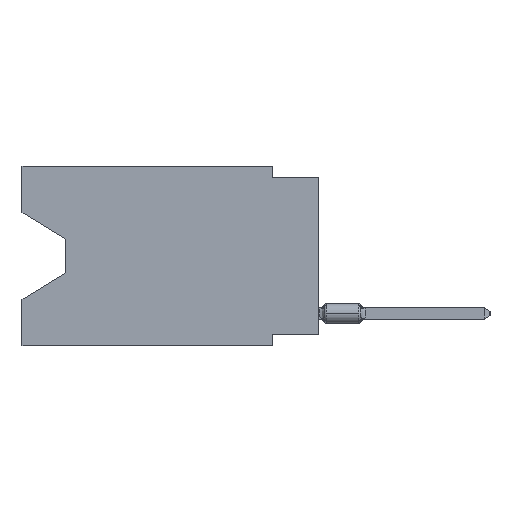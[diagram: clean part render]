
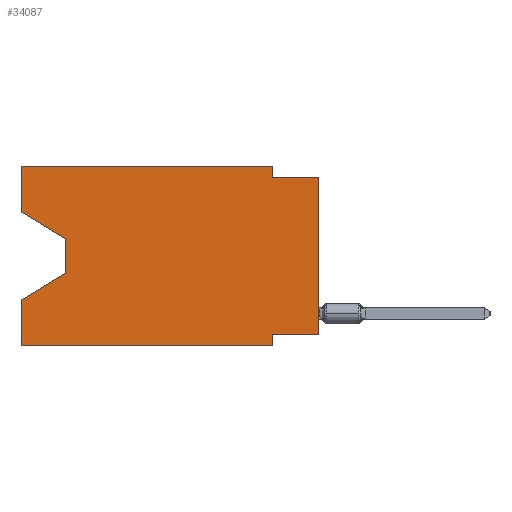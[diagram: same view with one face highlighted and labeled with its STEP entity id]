
A CAD part, left-side view. The second image highlights one B-rep face of the part: STEP entity #34087.
In plain terms, the highlighted planar face has unit normal (-1, 0, 0).
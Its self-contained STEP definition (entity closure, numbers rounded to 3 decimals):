
#524 = VERTEX_POINT ( 'NONE', #874 ) ;
#874 = CARTESIAN_POINT ( 'NONE',  ( 0., 2.54, -9.271 ) ) ;
#1854 = LINE ( 'NONE', #14686, #39917 ) ;
#3191 = FACE_OUTER_BOUND ( 'NONE', #37028, .T. ) ;
#3282 = VERTEX_POINT ( 'NONE', #44641 ) ;
#3413 = CARTESIAN_POINT ( 'NONE',  ( 0., 0., -9.271 ) ) ;
#3425 = VERTEX_POINT ( 'NONE', #6383 ) ;
#3441 = ORIENTED_EDGE ( 'NONE', *, *, #35888, .F. ) ;
#3469 = CARTESIAN_POINT ( 'NONE',  ( 0., 16.383, 0. ) ) ;
#4179 = VECTOR ( 'NONE', #18188, 1000. ) ;
#4365 = ORIENTED_EDGE ( 'NONE', *, *, #12885, .F. ) ;
#5211 = DIRECTION ( 'NONE',  ( 0., 0., 1. ) ) ;
#5479 = CARTESIAN_POINT ( 'NONE',  ( 0., 0., 0. ) ) ;
#5643 = LINE ( 'NONE', #26942, #4179 ) ;
#5719 = ORIENTED_EDGE ( 'NONE', *, *, #15789, .T. ) ;
#6383 = CARTESIAN_POINT ( 'NONE',  ( 0., 16.383, -2.546 ) ) ;
#6594 = ORIENTED_EDGE ( 'NONE', *, *, #8241, .F. ) ;
#6657 = DIRECTION ( 'NONE',  ( 0., 0., -1. ) ) ;
#7640 = CARTESIAN_POINT ( 'NONE',  ( 0., 13.97, -5.893 ) ) ;
#7889 = VECTOR ( 'NONE', #5211, 1000. ) ;
#8241 = EDGE_CURVE ( 'NONE', #13669, #27437, #14014, .T. ) ;
#9284 = VECTOR ( 'NONE', #46920, 1000. ) ;
#10106 = LINE ( 'NONE', #5479, #9284 ) ;
#10117 = LINE ( 'NONE', #22416, #7889 ) ;
#10159 = LINE ( 'NONE', #26845, #22671 ) ;
#10287 = VERTEX_POINT ( 'NONE', #7640 ) ;
#10940 = VECTOR ( 'NONE', #15010, 1000. ) ;
#11008 = ORIENTED_EDGE ( 'NONE', *, *, #31252, .F. ) ;
#11372 = EDGE_CURVE ( 'NONE', #49184, #30886, #10117, .T. ) ;
#11558 = CARTESIAN_POINT ( 'NONE',  ( 0., 2.54, 0. ) ) ;
#11641 = CARTESIAN_POINT ( 'NONE',  ( 0., 2.54, -0.635 ) ) ;
#12885 = EDGE_CURVE ( 'NONE', #27437, #40068, #23904, .T. ) ;
#13579 = CARTESIAN_POINT ( 'NONE',  ( 0., 13.97, -4.013 ) ) ;
#13669 = VERTEX_POINT ( 'NONE', #53870 ) ;
#14014 = LINE ( 'NONE', #11558, #39491 ) ;
#14410 = DIRECTION ( 'NONE',  ( 0., 0.855, -0.519 ) ) ;
#14686 = CARTESIAN_POINT ( 'NONE',  ( 0., 13.97, -5.893 ) ) ;
#15010 = DIRECTION ( 'NONE',  ( 0., -1., 0. ) ) ;
#15322 = EDGE_CURVE ( 'NONE', #33031, #40068, #10106, .T. ) ;
#15789 = EDGE_CURVE ( 'NONE', #10287, #30886, #1854, .T. ) ;
#17598 = ORIENTED_EDGE ( 'NONE', *, *, #26671, .F. ) ;
#17876 = CARTESIAN_POINT ( 'NONE',  ( 0., 0., -9.271 ) ) ;
#18188 = DIRECTION ( 'NONE',  ( 0., 0., 1. ) ) ;
#19279 = DIRECTION ( 'NONE',  ( 0., 1., 0. ) ) ;
#21974 = VECTOR ( 'NONE', #50192, 1000. ) ;
#22416 = CARTESIAN_POINT ( 'NONE',  ( 0., 16.383, 0. ) ) ;
#22671 = VECTOR ( 'NONE', #36095, 1000. ) ;
#22912 = VECTOR ( 'NONE', #19279, 1000. ) ;
#23423 = DIRECTION ( 'NONE',  ( 1., 0., 0. ) ) ;
#23904 = LINE ( 'NONE', #48677, #21974 ) ;
#24089 = VECTOR ( 'NONE', #6657, 1000. ) ;
#24423 = CARTESIAN_POINT ( 'NONE',  ( 0., 16.383, -2.546 ) ) ;
#24949 = LINE ( 'NONE', #24423, #40384 ) ;
#25768 = VERTEX_POINT ( 'NONE', #30425 ) ;
#26671 = EDGE_CURVE ( 'NONE', #3282, #13669, #39004, .T. ) ;
#26845 = CARTESIAN_POINT ( 'NONE',  ( 0., 16.383, -9.906 ) ) ;
#26942 = CARTESIAN_POINT ( 'NONE',  ( 0., 16.383, 0. ) ) ;
#27437 = VERTEX_POINT ( 'NONE', #11641 ) ;
#27722 = EDGE_CURVE ( 'NONE', #3425, #3282, #5643, .T. ) ;
#28751 = AXIS2_PLACEMENT_3D ( 'NONE', #3469, #23423, #49273 ) ;
#30425 = CARTESIAN_POINT ( 'NONE',  ( 0., 2.54, -9.906 ) ) ;
#30886 = VERTEX_POINT ( 'NONE', #50767 ) ;
#31224 = CARTESIAN_POINT ( 'NONE',  ( 0., 2.54, -9.906 ) ) ;
#31252 = EDGE_CURVE ( 'NONE', #524, #25768, #47571, .T. ) ;
#31376 = CARTESIAN_POINT ( 'NONE',  ( 0., 16.383, 0. ) ) ;
#32681 = ORIENTED_EDGE ( 'NONE', *, *, #15322, .T. ) ;
#33031 = VERTEX_POINT ( 'NONE', #17876 ) ;
#33451 = ORIENTED_EDGE ( 'NONE', *, *, #52516, .T. ) ;
#33745 = ORIENTED_EDGE ( 'NONE', *, *, #34375, .T. ) ;
#34087 = ADVANCED_FACE ( 'NONE', ( #3191 ), #40580, .F. ) ;
#34324 = LINE ( 'NONE', #13579, #36745 ) ;
#34375 = EDGE_CURVE ( 'NONE', #49184, #25768, #10159, .T. ) ;
#35120 = EDGE_CURVE ( 'NONE', #37663, #10287, #34324, .T. ) ;
#35888 = EDGE_CURVE ( 'NONE', #33031, #524, #52485, .T. ) ;
#36095 = DIRECTION ( 'NONE',  ( 0., -1., 0. ) ) ;
#36745 = VECTOR ( 'NONE', #42778, 1000. ) ;
#37028 = EDGE_LOOP ( 'NONE', ( #33451, #48163, #5719, #46350, #33745, #11008, #3441, #32681, #4365, #6594, #17598, #42446 ) ) ;
#37663 = VERTEX_POINT ( 'NONE', #50927 ) ;
#39004 = LINE ( 'NONE', #31376, #10940 ) ;
#39491 = VECTOR ( 'NONE', #40212, 1000. ) ;
#39873 = CARTESIAN_POINT ( 'NONE',  ( 0., 0., -0.635 ) ) ;
#39917 = VECTOR ( 'NONE', #14410, 1000. ) ;
#40068 = VERTEX_POINT ( 'NONE', #39873 ) ;
#40212 = DIRECTION ( 'NONE',  ( 0., 0., -1. ) ) ;
#40384 = VECTOR ( 'NONE', #49455, 1000. ) ;
#40580 = PLANE ( 'NONE',  #28751 ) ;
#42446 = ORIENTED_EDGE ( 'NONE', *, *, #27722, .F. ) ;
#42778 = DIRECTION ( 'NONE',  ( 0., 0., -1. ) ) ;
#44641 = CARTESIAN_POINT ( 'NONE',  ( 0., 16.383, 0. ) ) ;
#46350 = ORIENTED_EDGE ( 'NONE', *, *, #11372, .F. ) ;
#46920 = DIRECTION ( 'NONE',  ( 0., 0., 1. ) ) ;
#47571 = LINE ( 'NONE', #31224, #24089 ) ;
#48163 = ORIENTED_EDGE ( 'NONE', *, *, #35120, .T. ) ;
#48677 = CARTESIAN_POINT ( 'NONE',  ( 0., 0., -0.635 ) ) ;
#49184 = VERTEX_POINT ( 'NONE', #53096 ) ;
#49273 = DIRECTION ( 'NONE',  ( 0., 0., -1. ) ) ;
#49455 = DIRECTION ( 'NONE',  ( 0., -0.855, -0.519 ) ) ;
#50192 = DIRECTION ( 'NONE',  ( 0., -1., 0. ) ) ;
#50767 = CARTESIAN_POINT ( 'NONE',  ( 0., 16.383, -7.36 ) ) ;
#50927 = CARTESIAN_POINT ( 'NONE',  ( 0., 13.97, -4.013 ) ) ;
#52485 = LINE ( 'NONE', #3413, #22912 ) ;
#52516 = EDGE_CURVE ( 'NONE', #3425, #37663, #24949, .T. ) ;
#53096 = CARTESIAN_POINT ( 'NONE',  ( 0., 16.383, -9.906 ) ) ;
#53870 = CARTESIAN_POINT ( 'NONE',  ( 0., 2.54, 0. ) ) ;
